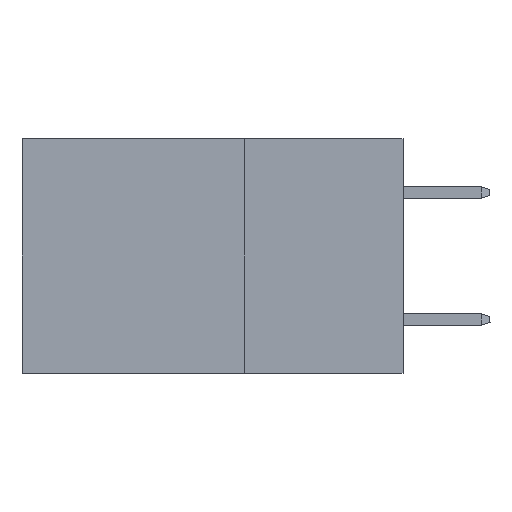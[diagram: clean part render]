
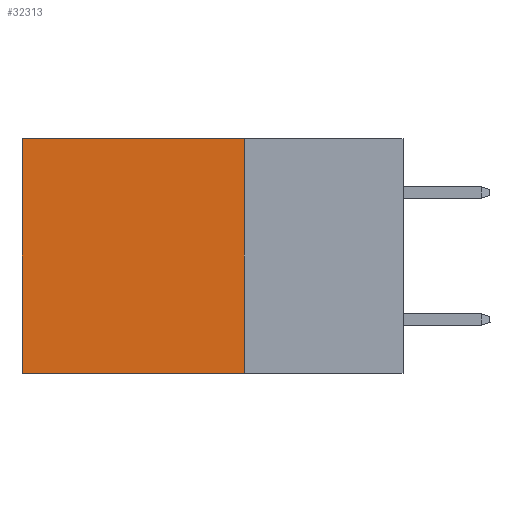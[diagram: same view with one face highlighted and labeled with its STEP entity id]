
A CAD part, left-side view. The second image highlights one B-rep face of the part: STEP entity #32313.
In plain terms, the highlighted planar face has unit normal (-1, 0, 0).
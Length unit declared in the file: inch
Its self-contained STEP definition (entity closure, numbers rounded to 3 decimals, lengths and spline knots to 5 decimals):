
#852 = CARTESIAN_POINT ( 'NONE',  ( 0.2875, 0.25, 0. ) ) ;
#2835 = VECTOR ( 'NONE', #37441, 39.37008 ) ;
#3953 = CARTESIAN_POINT ( 'NONE',  ( 0.2875, 0.6, -0.37 ) ) ;
#4761 = ORIENTED_EDGE ( 'NONE', *, *, #24535, .F. ) ;
#4800 = CARTESIAN_POINT ( 'NONE',  ( 0.2875, 0.25, -0.37 ) ) ;
#5026 = DIRECTION ( 'NONE',  ( 0., 1., 0. ) ) ;
#5220 = AXIS2_PLACEMENT_3D ( 'NONE', #14081, #35600, #28188 ) ;
#10733 = FACE_OUTER_BOUND ( 'NONE', #14271, .T. ) ;
#11922 = CARTESIAN_POINT ( 'NONE',  ( 0.2875, 0.6, 0. ) ) ;
#14081 = CARTESIAN_POINT ( 'NONE',  ( 0.2875, 0.25, 0. ) ) ;
#14271 = EDGE_LOOP ( 'NONE', ( #33278, #17369, #4761, #33695 ) ) ;
#16691 = CARTESIAN_POINT ( 'NONE',  ( 0.2875, 0.25, 0. ) ) ;
#17369 = ORIENTED_EDGE ( 'NONE', *, *, #28839, .F. ) ;
#19970 = EDGE_CURVE ( 'NONE', #41506, #24461, #33459, .T. ) ;
#20163 = CARTESIAN_POINT ( 'NONE',  ( 0.2875, 0.6, 0. ) ) ;
#21173 = CARTESIAN_POINT ( 'NONE',  ( 0.2875, 0.25, 0. ) ) ;
#21509 = VERTEX_POINT ( 'NONE', #42971 ) ;
#24461 = VERTEX_POINT ( 'NONE', #3953 ) ;
#24535 = EDGE_CURVE ( 'NONE', #39812, #21509, #44138, .T. ) ;
#27925 = LINE ( 'NONE', #16691, #39954 ) ;
#28188 = DIRECTION ( 'NONE',  ( 0., 0., -1. ) ) ;
#28839 = EDGE_CURVE ( 'NONE', #21509, #24461, #37803, .T. ) ;
#32313 = ADVANCED_FACE ( 'NONE', ( #10733 ), #39935, .F. ) ;
#33224 = DIRECTION ( 'NONE',  ( 0., 0., -1. ) ) ;
#33278 = ORIENTED_EDGE ( 'NONE', *, *, #19970, .T. ) ;
#33459 = LINE ( 'NONE', #11922, #37837 ) ;
#33695 = ORIENTED_EDGE ( 'NONE', *, *, #37990, .T. ) ;
#35600 = DIRECTION ( 'NONE',  ( 1., 0., 0. ) ) ;
#37441 = DIRECTION ( 'NONE',  ( 0., 0., -1. ) ) ;
#37803 = LINE ( 'NONE', #4800, #45597 ) ;
#37837 = VECTOR ( 'NONE', #33224, 39.37008 ) ;
#37990 = EDGE_CURVE ( 'NONE', #39812, #41506, #27925, .T. ) ;
#39812 = VERTEX_POINT ( 'NONE', #21173 ) ;
#39935 = PLANE ( 'NONE',  #5220 ) ;
#39954 = VECTOR ( 'NONE', #42996, 39.37008 ) ;
#41506 = VERTEX_POINT ( 'NONE', #20163 ) ;
#42971 = CARTESIAN_POINT ( 'NONE',  ( 0.2875, 0.25, -0.37 ) ) ;
#42996 = DIRECTION ( 'NONE',  ( 0., 1., 0. ) ) ;
#44138 = LINE ( 'NONE', #852, #2835 ) ;
#45597 = VECTOR ( 'NONE', #5026, 39.37008 ) ;
